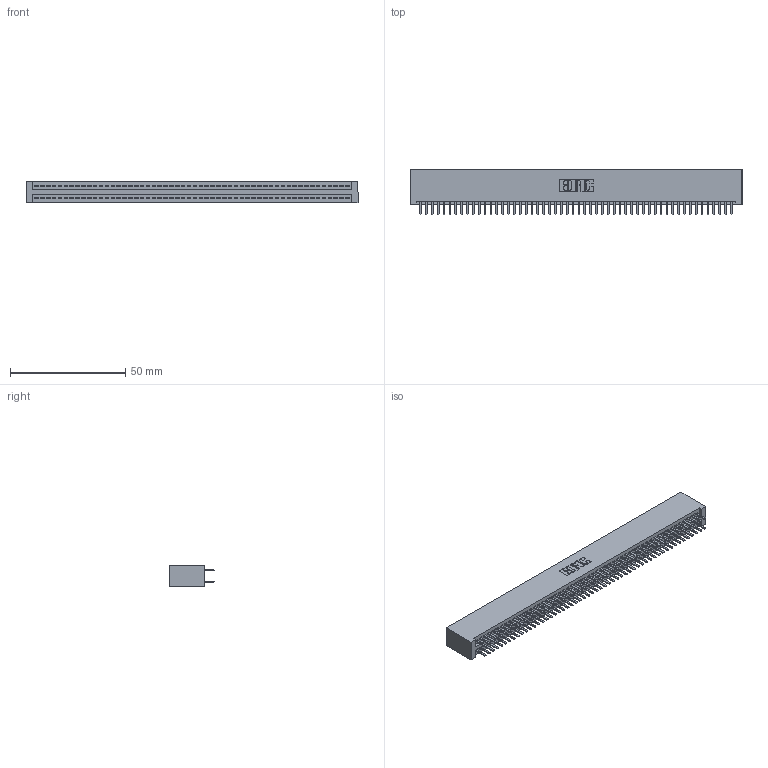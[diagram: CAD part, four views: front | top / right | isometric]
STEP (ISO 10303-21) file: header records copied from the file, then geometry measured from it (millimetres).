
FILE_DESCRIPTION (( 'STEP AP203' ), '1' );
FILE_NAME ('345-108-520-201.STEP', '2018-10-07T04:53:14', ( '' ), ( '' ), 'SwSTEP 2.0', 'SolidWorks 2016', '' );
FILE_SCHEMA (( 'CONFIG_CONTROL_DESIGN' ));
Length unit declared in the file: inch
Products named in the file (3): 345 Part_No Mounting Lugs; 345-292-001_345-293-120; 345-108-520-201
Assembly tree (109 placements, depth 2):
  345-108-520-201
    345 Part_No Mounting Lugs
    345-292-001_345-293-120  x108
Bounding box: 143.76 x 19.68 x 9.4 mm (x, y, z)
Volume: 14645.2 mm3; surface area: 22082.8 mm2
Topology: 109 solids, 109 shells, 5950 faces, 17273 edges, 11226 vertices
Faces by surface type: plane 3856, cylinder 2094
Entity records: 40591 total; most frequent: CARTESIAN_POINT 6804, ORIENTED_EDGE 6726, DIRECTION 5967, EDGE_CURVE 3363, LINE 3019, VECTOR 3019, VERTEX_POINT 2238, AXIS2_PLACEMENT_3D 1474
